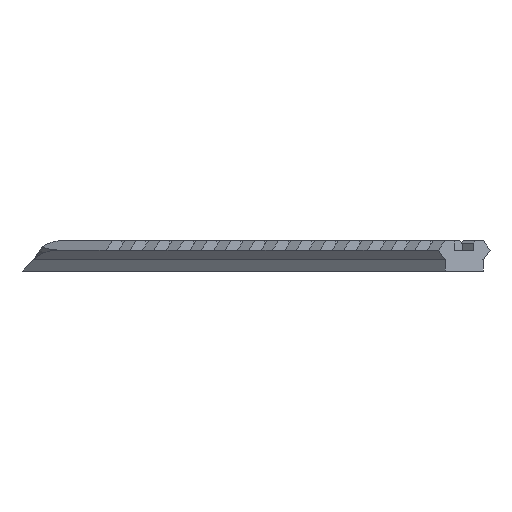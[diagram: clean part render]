
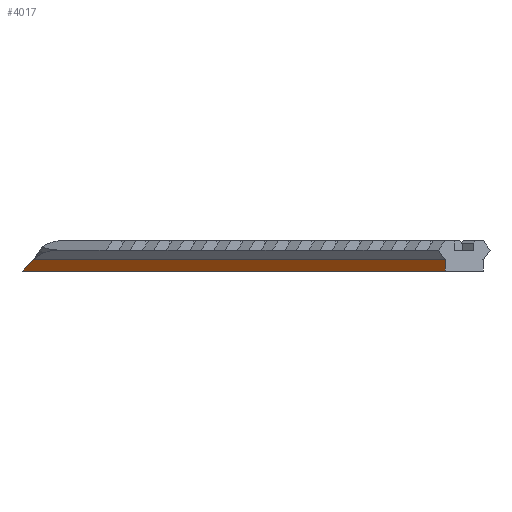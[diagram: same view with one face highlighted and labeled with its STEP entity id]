
A CAD part, front view. The second image highlights one B-rep face of the part: STEP entity #4017.
In plain terms, the highlighted planar face has unit normal (-0.707, -0.707, 0).
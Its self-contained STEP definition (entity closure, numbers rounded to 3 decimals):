
#54=PLANE('',#4271);
#254=FACE_OUTER_BOUND('',#470,.T.);
#470=EDGE_LOOP('',(#2883,#2884,#2885,#2886));
#667=LINE('',#5525,#1224);
#690=LINE('',#5637,#1247);
#691=LINE('',#5650,#1248);
#692=LINE('',#5651,#1249);
#1224=VECTOR('',#4477,10.);
#1247=VECTOR('',#4590,10.);
#1248=VECTOR('',#4603,10.);
#1249=VECTOR('',#4604,10.);
#1809=VERTEX_POINT('',#5522);
#1810=VERTEX_POINT('',#5524);
#1846=VERTEX_POINT('',#5635);
#1852=VERTEX_POINT('',#5649);
#2206=EDGE_CURVE('',#1810,#1809,#667,.T.);
#2257=EDGE_CURVE('',#1809,#1846,#690,.T.);
#2263=EDGE_CURVE('',#1852,#1846,#691,.T.);
#2264=EDGE_CURVE('',#1810,#1852,#692,.T.);
#2883=ORIENTED_EDGE('',*,*,#2257,.T.);
#2884=ORIENTED_EDGE('',*,*,#2263,.F.);
#2885=ORIENTED_EDGE('',*,*,#2264,.F.);
#2886=ORIENTED_EDGE('',*,*,#2206,.T.);
#4017=ADVANCED_FACE('',(#254),#54,.T.);
#4271=AXIS2_PLACEMENT_3D('',#5648,#4601,#4602);
#4477=DIRECTION('',(-0.58,0.58,-0.572));
#4590=DIRECTION('',(0.707,-0.707,0.));
#4601=DIRECTION('center_axis',(-0.707,-0.707,0.));
#4602=DIRECTION('ref_axis',(0.,0.,-1.));
#4603=DIRECTION('',(0.,0.,-1.));
#4604=DIRECTION('',(0.707,-0.707,0.));
#5522=CARTESIAN_POINT('',(-3.206,252.527,151.162));
#5524=CARTESIAN_POINT('',(0.355,248.966,154.672));
#5525=CARTESIAN_POINT('',(-10.057,259.379,144.407));
#5635=CARTESIAN_POINT('',(122.883,126.439,151.162));
#5637=CARTESIAN_POINT('',(53.687,195.635,151.162));
#5648=CARTESIAN_POINT('Origin',(-18.538,267.86,154.672));
#5649=CARTESIAN_POINT('',(122.883,126.439,154.672));
#5650=CARTESIAN_POINT('',(122.883,126.439,154.045));
#5651=CARTESIAN_POINT('',(115.812,133.51,154.672));
